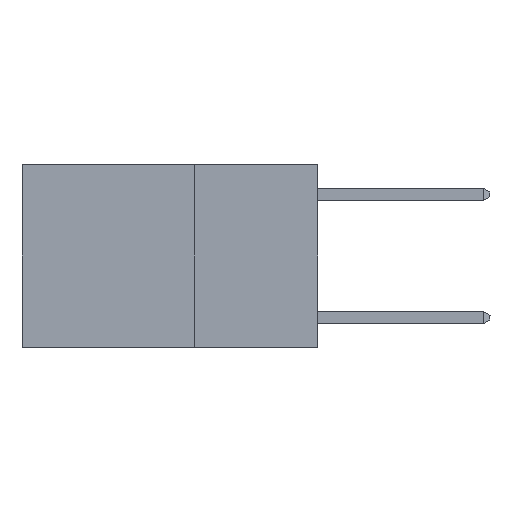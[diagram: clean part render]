
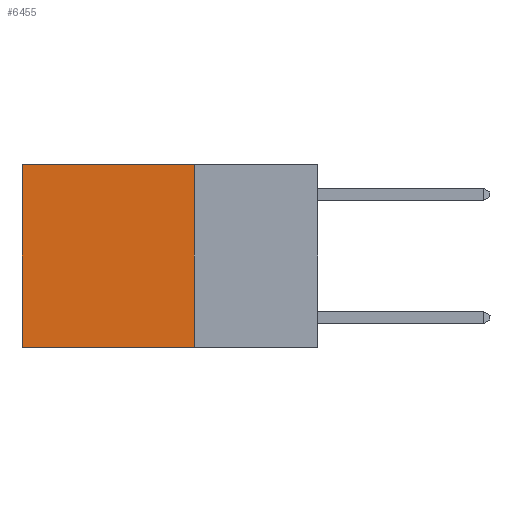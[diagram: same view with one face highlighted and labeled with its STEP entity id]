
A CAD part, left-side view. The second image highlights one B-rep face of the part: STEP entity #6455.
In plain terms, the highlighted planar face has unit normal (-1, 0, 0).
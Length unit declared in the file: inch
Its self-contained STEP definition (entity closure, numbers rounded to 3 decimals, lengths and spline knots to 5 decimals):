
#27 = PLANE ( 'NONE',  #9849 ) ;
#1070 = DIRECTION ( 'NONE',  ( 0., 1., 0. ) ) ;
#1571 = ORIENTED_EDGE ( 'NONE', *, *, #10907, .T. ) ;
#1820 = DIRECTION ( 'NONE',  ( 0., 0., -1. ) ) ;
#2512 = ORIENTED_EDGE ( 'NONE', *, *, #4933, .F. ) ;
#2767 = VECTOR ( 'NONE', #8452, 39.37008 ) ;
#2901 = VECTOR ( 'NONE', #8295, 39.37008 ) ;
#3527 = EDGE_LOOP ( 'NONE', ( #1571, #2512, #6310, #6535 ) ) ;
#3690 = CARTESIAN_POINT ( 'NONE',  ( 0.2625, 0.25, -0.37 ) ) ;
#4382 = VERTEX_POINT ( 'NONE', #7340 ) ;
#4933 = EDGE_CURVE ( 'NONE', #10898, #9281, #11034, .T. ) ;
#5203 = EDGE_CURVE ( 'NONE', #4382, #10898, #5276, .T. ) ;
#5274 = LINE ( 'NONE', #9275, #2901 ) ;
#5276 = LINE ( 'NONE', #5881, #2767 ) ;
#5881 = CARTESIAN_POINT ( 'NONE',  ( 0.2625, 0.25, 0. ) ) ;
#6310 = ORIENTED_EDGE ( 'NONE', *, *, #5203, .F. ) ;
#6455 = ADVANCED_FACE ( 'NONE', ( #11269 ), #27, .F. ) ;
#6520 = CARTESIAN_POINT ( 'NONE',  ( 0.2625, 0.25, 0. ) ) ;
#6535 = ORIENTED_EDGE ( 'NONE', *, *, #7244, .T. ) ;
#6759 = VECTOR ( 'NONE', #8208, 39.37008 ) ;
#6829 = VECTOR ( 'NONE', #1070, 39.37008 ) ;
#7086 = VERTEX_POINT ( 'NONE', #9936 ) ;
#7244 = EDGE_CURVE ( 'NONE', #4382, #7086, #7456, .T. ) ;
#7340 = CARTESIAN_POINT ( 'NONE',  ( 0.2625, 0.25, 0. ) ) ;
#7456 = LINE ( 'NONE', #6520, #6759 ) ;
#7964 = CARTESIAN_POINT ( 'NONE',  ( 0.2625, 0.25, 0. ) ) ;
#8208 = DIRECTION ( 'NONE',  ( 0., 1., 0. ) ) ;
#8295 = DIRECTION ( 'NONE',  ( 0., 0., -1. ) ) ;
#8452 = DIRECTION ( 'NONE',  ( 0., 0., -1. ) ) ;
#8678 = DIRECTION ( 'NONE',  ( 1., 0., 0. ) ) ;
#9275 = CARTESIAN_POINT ( 'NONE',  ( 0.2625, 0.6, 0. ) ) ;
#9281 = VERTEX_POINT ( 'NONE', #10449 ) ;
#9849 = AXIS2_PLACEMENT_3D ( 'NONE', #7964, #8678, #1820 ) ;
#9936 = CARTESIAN_POINT ( 'NONE',  ( 0.2625, 0.6, 0. ) ) ;
#10449 = CARTESIAN_POINT ( 'NONE',  ( 0.2625, 0.6, -0.37 ) ) ;
#10898 = VERTEX_POINT ( 'NONE', #11007 ) ;
#10907 = EDGE_CURVE ( 'NONE', #7086, #9281, #5274, .T. ) ;
#11007 = CARTESIAN_POINT ( 'NONE',  ( 0.2625, 0.25, -0.37 ) ) ;
#11034 = LINE ( 'NONE', #3690, #6829 ) ;
#11269 = FACE_OUTER_BOUND ( 'NONE', #3527, .T. ) ;
